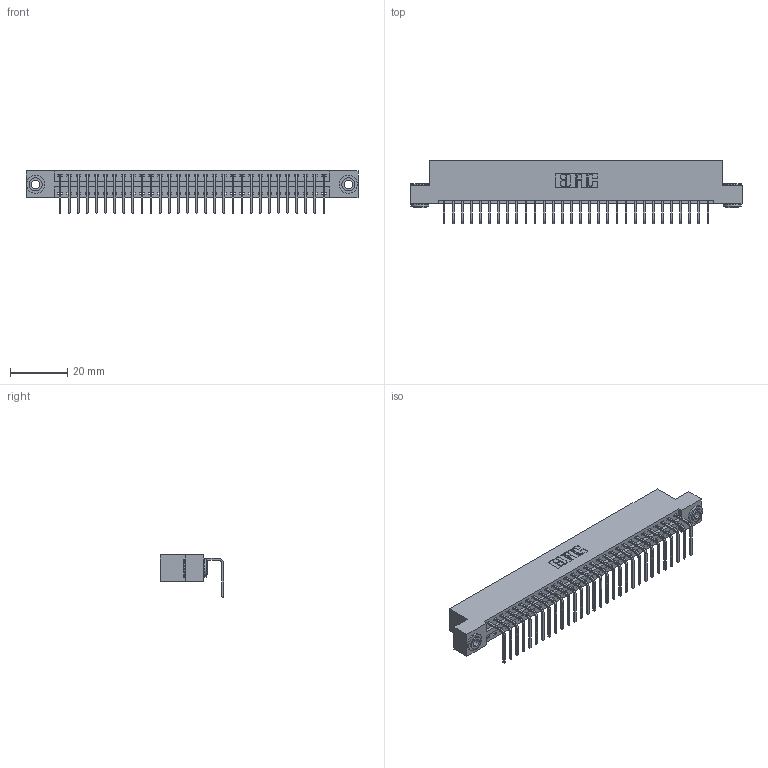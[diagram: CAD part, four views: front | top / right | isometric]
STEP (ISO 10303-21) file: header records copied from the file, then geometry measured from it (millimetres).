
FILE_DESCRIPTION (( 'STEP AP203' ), '1' );
FILE_NAME ('346-030-558-103.STEP', '2022-05-06T16:04:36', ( '' ), ( '' ), 'SwSTEP 2.0', 'SolidWorks 2020', '' );
FILE_SCHEMA (( 'CONFIG_CONTROL_DESIGN' ));
Length unit declared in the file: inch
Products named in the file (4): 346 Part_Flush Mounting Lugs - 0.156 Dia-TH; 346-030-558-103; 345-292-001_558 Tail - 2; 345-250-002_345-250-002-102
Assembly tree (33 placements, depth 2):
  346-030-558-103
    346 Part_Flush Mounting Lugs - 0.156 Dia-TH
    345-292-001_558 Tail - 2  x30
    345-250-002_345-250-002-102  x2
Bounding box: 115.82 x 22.16 x 14.73 mm (x, y, z)
Volume: 11105.5 mm3; surface area: 14598.7 mm2
Topology: 33 solids, 33 shells, 1974 faces, 5901 edges, 3890 vertices
Faces by surface type: plane 1360, cylinder 606, cone 8
Entity records: 21384 total; most frequent: CARTESIAN_POINT 3651, ORIENTED_EDGE 3606, DIRECTION 3265, EDGE_CURVE 1803, LINE 1527, VECTOR 1527, VERTEX_POINT 1198, AXIS2_PLACEMENT_3D 869
